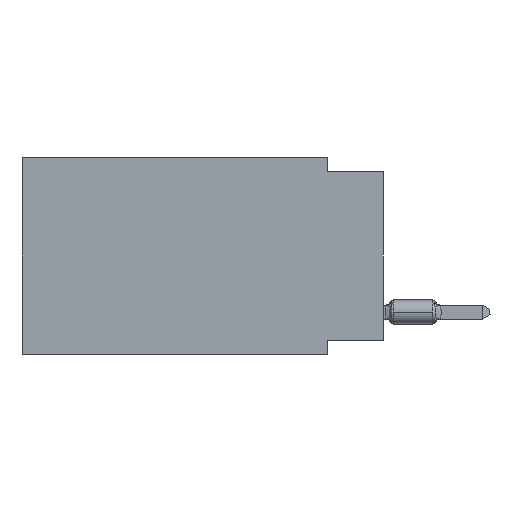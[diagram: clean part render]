
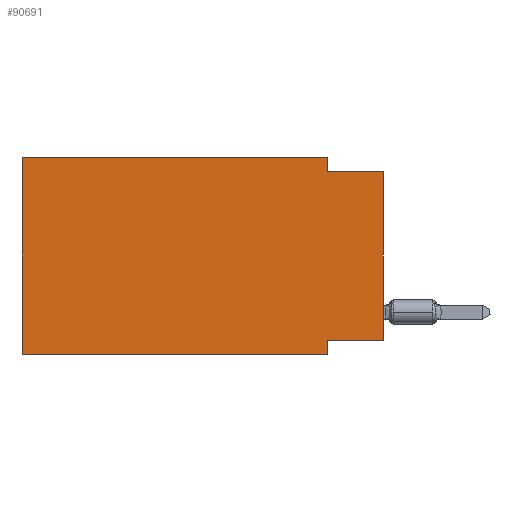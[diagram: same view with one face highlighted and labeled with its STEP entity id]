
A CAD part, left-side view. The second image highlights one B-rep face of the part: STEP entity #90691.
In plain terms, the highlighted planar face has unit normal (-1, 0, 0).
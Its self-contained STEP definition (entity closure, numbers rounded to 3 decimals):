
#322 = LINE ( 'NONE', #78110, #68660 ) ;
#573 = VERTEX_POINT ( 'NONE', #90762 ) ;
#2169 = CARTESIAN_POINT ( 'NONE',  ( 0., 0., 0. ) ) ;
#2350 = EDGE_CURVE ( 'NONE', #43533, #49143, #73828, .T. ) ;
#5752 = FACE_OUTER_BOUND ( 'NONE', #57810, .T. ) ;
#5894 = EDGE_CURVE ( 'NONE', #573, #23995, #16130, .T. ) ;
#6214 = PLANE ( 'NONE',  #38025 ) ;
#10037 = CARTESIAN_POINT ( 'NONE',  ( 0., 2.54, 0. ) ) ;
#10244 = CARTESIAN_POINT ( 'NONE',  ( 0., 2.54, -8.89 ) ) ;
#10975 = VERTEX_POINT ( 'NONE', #60138 ) ;
#11802 = DIRECTION ( 'NONE',  ( 0., 0., -1. ) ) ;
#11996 = CARTESIAN_POINT ( 'NONE',  ( 0., 0., -8.255 ) ) ;
#13010 = CARTESIAN_POINT ( 'NONE',  ( 0., 16.383, 0. ) ) ;
#13337 = EDGE_CURVE ( 'NONE', #49143, #23995, #322, .T. ) ;
#15726 = VERTEX_POINT ( 'NONE', #59055 ) ;
#16130 = LINE ( 'NONE', #2169, #53095 ) ;
#19771 = CARTESIAN_POINT ( 'NONE',  ( 0., 2.54, 0. ) ) ;
#22677 = ORIENTED_EDGE ( 'NONE', *, *, #82211, .F. ) ;
#23907 = ORIENTED_EDGE ( 'NONE', *, *, #49456, .F. ) ;
#23995 = VERTEX_POINT ( 'NONE', #72317 ) ;
#25986 = LINE ( 'NONE', #11996, #82565 ) ;
#28606 = ORIENTED_EDGE ( 'NONE', *, *, #81834, .T. ) ;
#30664 = VERTEX_POINT ( 'NONE', #61686 ) ;
#31560 = ORIENTED_EDGE ( 'NONE', *, *, #13337, .F. ) ;
#34631 = DIRECTION ( 'NONE',  ( 1., 0., 0. ) ) ;
#34936 = VECTOR ( 'NONE', #89194, 1000. ) ;
#37024 = EDGE_CURVE ( 'NONE', #30664, #53338, #84265, .T. ) ;
#37991 = DIRECTION ( 'NONE',  ( 0., 0., -1. ) ) ;
#38025 = AXIS2_PLACEMENT_3D ( 'NONE', #54654, #34631, #11802 ) ;
#43533 = VERTEX_POINT ( 'NONE', #19771 ) ;
#44178 = LINE ( 'NONE', #58155, #61620 ) ;
#45696 = EDGE_CURVE ( 'NONE', #53338, #43533, #44178, .T. ) ;
#46318 = VECTOR ( 'NONE', #60081, 1000. ) ;
#48860 = DIRECTION ( 'NONE',  ( 0., 0., 1. ) ) ;
#49143 = VERTEX_POINT ( 'NONE', #69943 ) ;
#49456 = EDGE_CURVE ( 'NONE', #10975, #15726, #74044, .T. ) ;
#50563 = ORIENTED_EDGE ( 'NONE', *, *, #2350, .F. ) ;
#51963 = DIRECTION ( 'NONE',  ( 0., 0., 1. ) ) ;
#53095 = VECTOR ( 'NONE', #51963, 1000. ) ;
#53119 = ORIENTED_EDGE ( 'NONE', *, *, #45696, .F. ) ;
#53338 = VERTEX_POINT ( 'NONE', #13010 ) ;
#54654 = CARTESIAN_POINT ( 'NONE',  ( 0., 16.383, 0. ) ) ;
#57141 = DIRECTION ( 'NONE',  ( 0., -1., 0. ) ) ;
#57248 = VECTOR ( 'NONE', #48860, 1000. ) ;
#57810 = EDGE_LOOP ( 'NONE', ( #85217, #31560, #50563, #53119, #77454, #28606, #23907, #22677 ) ) ;
#58155 = CARTESIAN_POINT ( 'NONE',  ( 0., 16.383, 0. ) ) ;
#59055 = CARTESIAN_POINT ( 'NONE',  ( 0., 2.54, -8.89 ) ) ;
#60081 = DIRECTION ( 'NONE',  ( 0., 0., -1. ) ) ;
#60138 = CARTESIAN_POINT ( 'NONE',  ( 0., 2.54, -8.255 ) ) ;
#61620 = VECTOR ( 'NONE', #84749, 1000. ) ;
#61686 = CARTESIAN_POINT ( 'NONE',  ( 0., 16.383, -8.89 ) ) ;
#61740 = CARTESIAN_POINT ( 'NONE',  ( 0., 16.383, -8.89 ) ) ;
#68660 = VECTOR ( 'NONE', #57141, 1000. ) ;
#69943 = CARTESIAN_POINT ( 'NONE',  ( 0., 2.54, -0.635 ) ) ;
#72317 = CARTESIAN_POINT ( 'NONE',  ( 0., 0., -0.635 ) ) ;
#73828 = LINE ( 'NONE', #10037, #82309 ) ;
#74044 = LINE ( 'NONE', #10244, #46318 ) ;
#77454 = ORIENTED_EDGE ( 'NONE', *, *, #37024, .F. ) ;
#78110 = CARTESIAN_POINT ( 'NONE',  ( 0., 0., -0.635 ) ) ;
#81834 = EDGE_CURVE ( 'NONE', #30664, #15726, #82230, .T. ) ;
#82211 = EDGE_CURVE ( 'NONE', #573, #10975, #25986, .T. ) ;
#82230 = LINE ( 'NONE', #61740, #34936 ) ;
#82309 = VECTOR ( 'NONE', #37991, 1000. ) ;
#82565 = VECTOR ( 'NONE', #89769, 1000. ) ;
#83313 = CARTESIAN_POINT ( 'NONE',  ( 0., 16.383, 0. ) ) ;
#84265 = LINE ( 'NONE', #83313, #57248 ) ;
#84749 = DIRECTION ( 'NONE',  ( 0., -1., 0. ) ) ;
#85217 = ORIENTED_EDGE ( 'NONE', *, *, #5894, .T. ) ;
#89194 = DIRECTION ( 'NONE',  ( 0., -1., 0. ) ) ;
#89769 = DIRECTION ( 'NONE',  ( 0., 1., 0. ) ) ;
#90691 = ADVANCED_FACE ( 'NONE', ( #5752 ), #6214, .F. ) ;
#90762 = CARTESIAN_POINT ( 'NONE',  ( 0., 0., -8.255 ) ) ;
